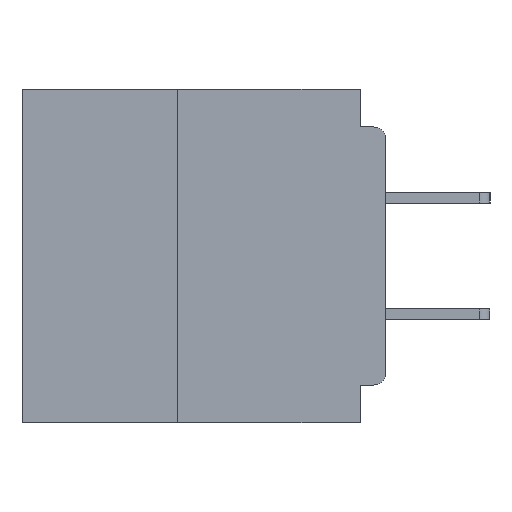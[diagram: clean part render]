
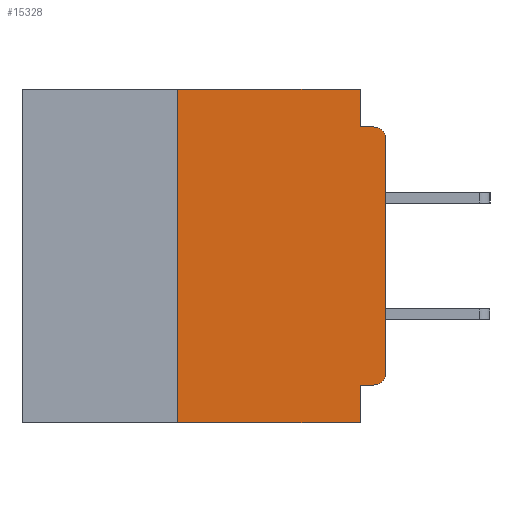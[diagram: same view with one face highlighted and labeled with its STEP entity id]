
A CAD part, left-side view. The second image highlights one B-rep face of the part: STEP entity #15328.
In plain terms, the highlighted planar face has unit normal (-1, 0, 0).
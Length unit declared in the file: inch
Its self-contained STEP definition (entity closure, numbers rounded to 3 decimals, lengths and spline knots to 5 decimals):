
#299 = CARTESIAN_POINT ( 'NONE',  ( 0., 0., 0. ) ) ;
#2509 = CARTESIAN_POINT ( 'NONE',  ( 0., 0.031, -0.4 ) ) ;
#2943 = FACE_OUTER_BOUND ( 'NONE', #51461, .T. ) ;
#3472 = VERTEX_POINT ( 'NONE', #21730 ) ;
#3888 = AXIS2_PLACEMENT_3D ( 'NONE', #27151, #59110, #31790 ) ;
#3890 = EDGE_CURVE ( 'NONE', #23593, #3472, #55633, .T. ) ;
#4082 = DIRECTION ( 'NONE',  ( 0., 0., -1. ) ) ;
#5172 = VERTEX_POINT ( 'NONE', #15727 ) ;
#5714 = AXIS2_PLACEMENT_3D ( 'NONE', #27067, #31707, #4082 ) ;
#7071 = ORIENTED_EDGE ( 'NONE', *, *, #12125, .F. ) ;
#7584 = CIRCLE ( 'NONE', #49266, 0.015 ) ;
#8230 = VECTOR ( 'NONE', #25430, 39.37008 ) ;
#8332 = EDGE_CURVE ( 'NONE', #58623, #19809, #54129, .T. ) ;
#11374 = LINE ( 'NONE', #26731, #34374 ) ;
#11441 = EDGE_CURVE ( 'NONE', #36603, #19809, #43839, .T. ) ;
#11568 = VECTOR ( 'NONE', #27912, 39.37008 ) ;
#12125 = EDGE_CURVE ( 'NONE', #16000, #5172, #57080, .T. ) ;
#12962 = ORIENTED_EDGE ( 'NONE', *, *, #3890, .F. ) ;
#13391 = CARTESIAN_POINT ( 'NONE',  ( 0., 0.25, 0. ) ) ;
#14711 = CARTESIAN_POINT ( 'NONE',  ( 0., 0.015, -0.355 ) ) ;
#15328 = ADVANCED_FACE ( 'NONE', ( #2943 ), #54449, .F. ) ;
#15727 = CARTESIAN_POINT ( 'NONE',  ( 0., 0.015, -0.045 ) ) ;
#16000 = VERTEX_POINT ( 'NONE', #22539 ) ;
#16925 = DIRECTION ( 'NONE',  ( 0., 1., 0. ) ) ;
#17146 = ORIENTED_EDGE ( 'NONE', *, *, #49418, .F. ) ;
#17671 = CARTESIAN_POINT ( 'NONE',  ( 0., 0., -0.34 ) ) ;
#19153 = VECTOR ( 'NONE', #35063, 39.37008 ) ;
#19809 = VERTEX_POINT ( 'NONE', #32382 ) ;
#21730 = CARTESIAN_POINT ( 'NONE',  ( 0., 0.031, 0. ) ) ;
#22539 = CARTESIAN_POINT ( 'NONE',  ( 0., 0.031, -0.045 ) ) ;
#23593 = VERTEX_POINT ( 'NONE', #13391 ) ;
#25430 = DIRECTION ( 'NONE',  ( 0., -1., 0. ) ) ;
#25579 = ORIENTED_EDGE ( 'NONE', *, *, #8332, .T. ) ;
#25644 = CARTESIAN_POINT ( 'NONE',  ( 0., 0.015, -0.34 ) ) ;
#26731 = CARTESIAN_POINT ( 'NONE',  ( 0., 0.25, -0.4 ) ) ;
#27067 = CARTESIAN_POINT ( 'NONE',  ( 0., 0.437, 0. ) ) ;
#27151 = CARTESIAN_POINT ( 'NONE',  ( 0., 0.015, -0.06 ) ) ;
#27229 = DIRECTION ( 'NONE',  ( 0., 0., -1. ) ) ;
#27912 = DIRECTION ( 'NONE',  ( 0., 0., 1. ) ) ;
#28717 = EDGE_CURVE ( 'NONE', #47654, #51552, #37433, .T. ) ;
#30308 = DIRECTION ( 'NONE',  ( 0., 0., -1. ) ) ;
#31356 = DIRECTION ( 'NONE',  ( 0., 0., 1. ) ) ;
#31707 = DIRECTION ( 'NONE',  ( 1., 0., 0. ) ) ;
#31715 = VECTOR ( 'NONE', #57491, 39.37008 ) ;
#31790 = DIRECTION ( 'NONE',  ( 0., 0., -1. ) ) ;
#32382 = CARTESIAN_POINT ( 'NONE',  ( 0., 0.031, -0.4 ) ) ;
#32642 = DIRECTION ( 'NONE',  ( 0., -1., 0. ) ) ;
#33714 = EDGE_CURVE ( 'NONE', #53937, #36603, #39860, .T. ) ;
#34374 = VECTOR ( 'NONE', #31356, 39.37008 ) ;
#35063 = DIRECTION ( 'NONE',  ( 0., -1., 0. ) ) ;
#36194 = VECTOR ( 'NONE', #27229, 39.37008 ) ;
#36401 = ORIENTED_EDGE ( 'NONE', *, *, #58177, .T. ) ;
#36603 = VERTEX_POINT ( 'NONE', #37965 ) ;
#37433 = LINE ( 'NONE', #299, #11568 ) ;
#37674 = CIRCLE ( 'NONE', #3888, 0.015 ) ;
#37965 = CARTESIAN_POINT ( 'NONE',  ( 0., 0.031, -0.355 ) ) ;
#38808 = CARTESIAN_POINT ( 'NONE',  ( 0., 0.437, 0. ) ) ;
#39636 = CARTESIAN_POINT ( 'NONE',  ( 0., 0., -0.045 ) ) ;
#39860 = LINE ( 'NONE', #58104, #50586 ) ;
#42537 = ORIENTED_EDGE ( 'NONE', *, *, #11441, .F. ) ;
#42808 = ORIENTED_EDGE ( 'NONE', *, *, #28717, .T. ) ;
#43490 = VECTOR ( 'NONE', #32642, 39.37008 ) ;
#43839 = LINE ( 'NONE', #2509, #31715 ) ;
#45177 = ORIENTED_EDGE ( 'NONE', *, *, #33714, .F. ) ;
#47654 = VERTEX_POINT ( 'NONE', #17671 ) ;
#48306 = LINE ( 'NONE', #50195, #36194 ) ;
#48972 = EDGE_CURVE ( 'NONE', #51552, #5172, #37674, .T. ) ;
#49266 = AXIS2_PLACEMENT_3D ( 'NONE', #25644, #57631, #30308 ) ;
#49418 = EDGE_CURVE ( 'NONE', #3472, #16000, #48306, .T. ) ;
#50195 = CARTESIAN_POINT ( 'NONE',  ( 0., 0.031, 0. ) ) ;
#50586 = VECTOR ( 'NONE', #16925, 39.37008 ) ;
#51461 = EDGE_LOOP ( 'NONE', ( #42808, #53696, #7071, #17146, #12962, #52195, #25579, #42537, #45177, #36401 ) ) ;
#51552 = VERTEX_POINT ( 'NONE', #51739 ) ;
#51739 = CARTESIAN_POINT ( 'NONE',  ( 0., 0., -0.06 ) ) ;
#52195 = ORIENTED_EDGE ( 'NONE', *, *, #52493, .F. ) ;
#52397 = CARTESIAN_POINT ( 'NONE',  ( 0., 0.25, -0.4 ) ) ;
#52493 = EDGE_CURVE ( 'NONE', #58623, #23593, #11374, .T. ) ;
#52830 = CARTESIAN_POINT ( 'NONE',  ( 0., 0.437, -0.4 ) ) ;
#53696 = ORIENTED_EDGE ( 'NONE', *, *, #48972, .T. ) ;
#53937 = VERTEX_POINT ( 'NONE', #14711 ) ;
#54129 = LINE ( 'NONE', #52830, #8230 ) ;
#54449 = PLANE ( 'NONE',  #5714 ) ;
#55633 = LINE ( 'NONE', #38808, #43490 ) ;
#57080 = LINE ( 'NONE', #39636, #19153 ) ;
#57491 = DIRECTION ( 'NONE',  ( 0., 0., -1. ) ) ;
#57631 = DIRECTION ( 'NONE',  ( -1., 0., 0. ) ) ;
#58104 = CARTESIAN_POINT ( 'NONE',  ( 0., 0., -0.355 ) ) ;
#58177 = EDGE_CURVE ( 'NONE', #53937, #47654, #7584, .T. ) ;
#58623 = VERTEX_POINT ( 'NONE', #52397 ) ;
#59110 = DIRECTION ( 'NONE',  ( -1., 0., 0. ) ) ;
